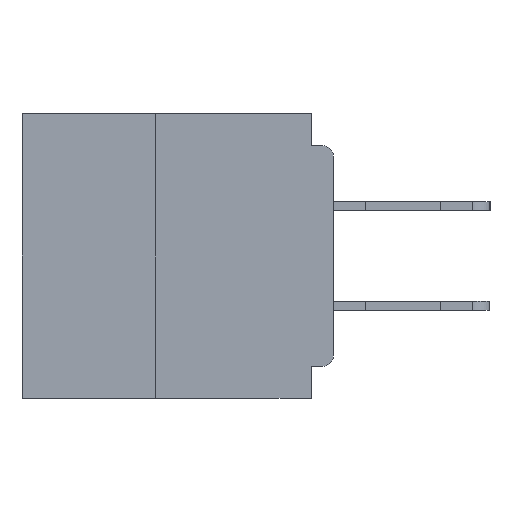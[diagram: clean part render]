
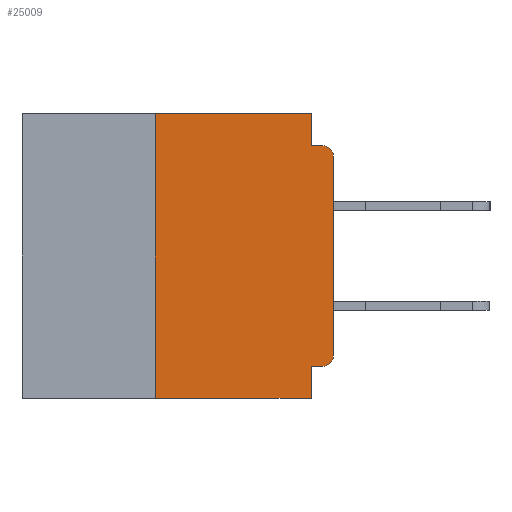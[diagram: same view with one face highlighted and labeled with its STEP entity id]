
A CAD part, left-side view. The second image highlights one B-rep face of the part: STEP entity #25009.
In plain terms, the highlighted planar face has unit normal (-1, 0, 0).
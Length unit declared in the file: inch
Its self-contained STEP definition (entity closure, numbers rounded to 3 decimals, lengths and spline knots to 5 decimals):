
#341 = ORIENTED_EDGE ( 'NONE', *, *, #18169, .F. ) ;
#903 = EDGE_LOOP ( 'NONE', ( #36782, #8554, #23739, #17173, #3543, #26365, #12229, #28143, #341, #23308 ) ) ;
#1363 = LINE ( 'NONE', #26528, #30872 ) ;
#2262 = VECTOR ( 'NONE', #13638, 39.37008 ) ;
#2381 = VERTEX_POINT ( 'NONE', #11627 ) ;
#2582 = AXIS2_PLACEMENT_3D ( 'NONE', #21009, #3807, #23854 ) ;
#2953 = VECTOR ( 'NONE', #25162, 39.37008 ) ;
#3471 = CARTESIAN_POINT ( 'NONE',  ( 0., 0.031, -0.045 ) ) ;
#3543 = ORIENTED_EDGE ( 'NONE', *, *, #27262, .F. ) ;
#3761 = VERTEX_POINT ( 'NONE', #14246 ) ;
#3807 = DIRECTION ( 'NONE',  ( -1., 0., 0. ) ) ;
#4002 = CARTESIAN_POINT ( 'NONE',  ( 0., 0., -0.355 ) ) ;
#4638 = VERTEX_POINT ( 'NONE', #3471 ) ;
#5890 = CARTESIAN_POINT ( 'NONE',  ( 0., 0.015, -0.045 ) ) ;
#5902 = VECTOR ( 'NONE', #23721, 39.37008 ) ;
#6495 = VERTEX_POINT ( 'NONE', #17994 ) ;
#6673 = CARTESIAN_POINT ( 'NONE',  ( 0., 0.015, -0.34 ) ) ;
#7415 = VECTOR ( 'NONE', #26983, 39.37008 ) ;
#8554 = ORIENTED_EDGE ( 'NONE', *, *, #34489, .T. ) ;
#9611 = DIRECTION ( 'NONE',  ( 0., 0., -1. ) ) ;
#10930 = CARTESIAN_POINT ( 'NONE',  ( 0., 0.031, -0.355 ) ) ;
#11428 = CARTESIAN_POINT ( 'NONE',  ( 0., 0.031, -0.4 ) ) ;
#11627 = CARTESIAN_POINT ( 'NONE',  ( 0., 0.25, -0.4 ) ) ;
#11836 = VECTOR ( 'NONE', #32314, 39.37008 ) ;
#11947 = CARTESIAN_POINT ( 'NONE',  ( 0., 0.437, 0. ) ) ;
#12229 = ORIENTED_EDGE ( 'NONE', *, *, #14176, .T. ) ;
#12248 = EDGE_CURVE ( 'NONE', #32594, #23104, #32627, .T. ) ;
#12675 = DIRECTION ( 'NONE',  ( 0., 1., 0. ) ) ;
#13197 = CARTESIAN_POINT ( 'NONE',  ( 0., 0., -0.34 ) ) ;
#13633 = AXIS2_PLACEMENT_3D ( 'NONE', #6673, #26608, #9611 ) ;
#13638 = DIRECTION ( 'NONE',  ( 0., 0., 1. ) ) ;
#14176 = EDGE_CURVE ( 'NONE', #2381, #19137, #18373, .T. ) ;
#14246 = CARTESIAN_POINT ( 'NONE',  ( 0., 0.031, 0. ) ) ;
#14857 = DIRECTION ( 'NONE',  ( 0., 0., -1. ) ) ;
#15165 = LINE ( 'NONE', #21318, #7415 ) ;
#15522 = VECTOR ( 'NONE', #22471, 39.37008 ) ;
#16266 = EDGE_CURVE ( 'NONE', #25565, #32594, #29191, .T. ) ;
#16741 = FACE_OUTER_BOUND ( 'NONE', #903, .T. ) ;
#17173 = ORIENTED_EDGE ( 'NONE', *, *, #17438, .F. ) ;
#17435 = AXIS2_PLACEMENT_3D ( 'NONE', #11947, #31690, #14857 ) ;
#17438 = EDGE_CURVE ( 'NONE', #3761, #4638, #29545, .T. ) ;
#17506 = EDGE_CURVE ( 'NONE', #4638, #23852, #33464, .T. ) ;
#17585 = PLANE ( 'NONE',  #17435 ) ;
#17994 = CARTESIAN_POINT ( 'NONE',  ( 0., 0.25, 0. ) ) ;
#18169 = EDGE_CURVE ( 'NONE', #25565, #30098, #25492, .T. ) ;
#18214 = DIRECTION ( 'NONE',  ( 0., -1., 0. ) ) ;
#18373 = LINE ( 'NONE', #30570, #2953 ) ;
#18567 = CARTESIAN_POINT ( 'NONE',  ( 0., 0.015, -0.355 ) ) ;
#19137 = VERTEX_POINT ( 'NONE', #11428 ) ;
#20879 = CARTESIAN_POINT ( 'NONE',  ( 0., 0.031, 0. ) ) ;
#21009 = CARTESIAN_POINT ( 'NONE',  ( 0., 0.015, -0.06 ) ) ;
#21318 = CARTESIAN_POINT ( 'NONE',  ( 0., 0.031, -0.4 ) ) ;
#22107 = LINE ( 'NONE', #36371, #15522 ) ;
#22471 = DIRECTION ( 'NONE',  ( 0., 0., 1. ) ) ;
#22484 = EDGE_CURVE ( 'NONE', #30098, #19137, #15165, .T. ) ;
#23104 = VERTEX_POINT ( 'NONE', #33647 ) ;
#23308 = ORIENTED_EDGE ( 'NONE', *, *, #16266, .T. ) ;
#23721 = DIRECTION ( 'NONE',  ( 0., 0., -1. ) ) ;
#23739 = ORIENTED_EDGE ( 'NONE', *, *, #17506, .F. ) ;
#23852 = VERTEX_POINT ( 'NONE', #5890 ) ;
#23854 = DIRECTION ( 'NONE',  ( 0., 0., -1. ) ) ;
#23964 = CARTESIAN_POINT ( 'NONE',  ( 0., 0., -0.045 ) ) ;
#25009 = ADVANCED_FACE ( 'NONE', ( #16741 ), #17585, .F. ) ;
#25162 = DIRECTION ( 'NONE',  ( 0., -1., 0. ) ) ;
#25492 = LINE ( 'NONE', #4002, #26373 ) ;
#25565 = VERTEX_POINT ( 'NONE', #18567 ) ;
#26365 = ORIENTED_EDGE ( 'NONE', *, *, #34825, .F. ) ;
#26373 = VECTOR ( 'NONE', #12675, 39.37008 ) ;
#26528 = CARTESIAN_POINT ( 'NONE',  ( 0., 0.437, 0. ) ) ;
#26608 = DIRECTION ( 'NONE',  ( -1., 0., 0. ) ) ;
#26983 = DIRECTION ( 'NONE',  ( 0., 0., -1. ) ) ;
#27262 = EDGE_CURVE ( 'NONE', #6495, #3761, #1363, .T. ) ;
#27698 = CARTESIAN_POINT ( 'NONE',  ( 0., 0., 0. ) ) ;
#28143 = ORIENTED_EDGE ( 'NONE', *, *, #22484, .F. ) ;
#29191 = CIRCLE ( 'NONE', #13633, 0.015 ) ;
#29545 = LINE ( 'NONE', #20879, #5902 ) ;
#30098 = VERTEX_POINT ( 'NONE', #10930 ) ;
#30570 = CARTESIAN_POINT ( 'NONE',  ( 0., 0.437, -0.4 ) ) ;
#30872 = VECTOR ( 'NONE', #18214, 39.37008 ) ;
#31690 = DIRECTION ( 'NONE',  ( 1., 0., 0. ) ) ;
#32314 = DIRECTION ( 'NONE',  ( 0., -1., 0. ) ) ;
#32594 = VERTEX_POINT ( 'NONE', #13197 ) ;
#32627 = LINE ( 'NONE', #27698, #2262 ) ;
#33464 = LINE ( 'NONE', #23964, #11836 ) ;
#33558 = CIRCLE ( 'NONE', #2582, 0.015 ) ;
#33647 = CARTESIAN_POINT ( 'NONE',  ( 0., 0., -0.06 ) ) ;
#34489 = EDGE_CURVE ( 'NONE', #23104, #23852, #33558, .T. ) ;
#34825 = EDGE_CURVE ( 'NONE', #2381, #6495, #22107, .T. ) ;
#36371 = CARTESIAN_POINT ( 'NONE',  ( 0., 0.25, -0.4 ) ) ;
#36782 = ORIENTED_EDGE ( 'NONE', *, *, #12248, .T. ) ;
